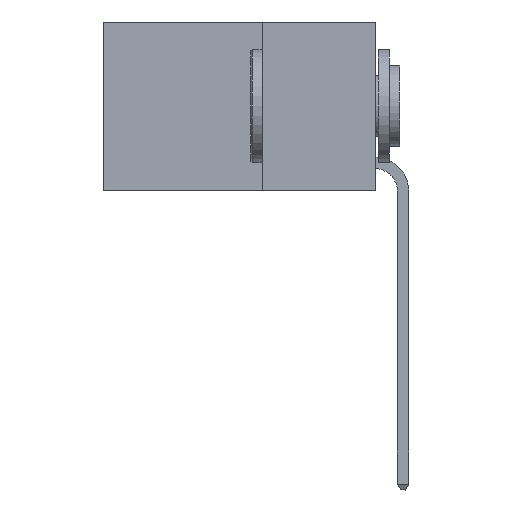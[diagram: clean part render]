
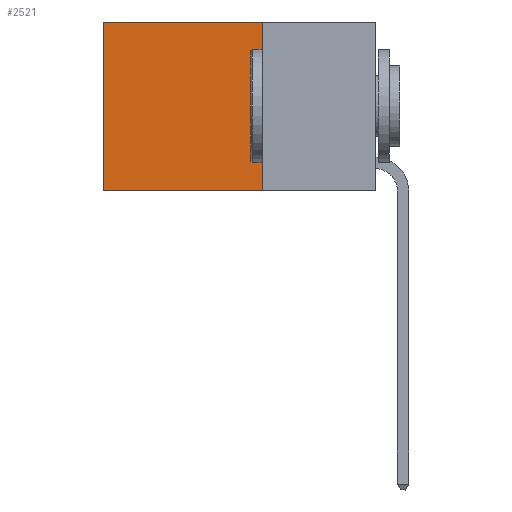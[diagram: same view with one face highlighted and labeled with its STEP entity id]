
A CAD part, left-side view. The second image highlights one B-rep face of the part: STEP entity #2521.
In plain terms, the highlighted planar face has unit normal (-1, 0, 0).
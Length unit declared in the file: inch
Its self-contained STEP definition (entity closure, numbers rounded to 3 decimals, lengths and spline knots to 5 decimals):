
#138 = DIRECTION ( 'NONE',  ( 1., 0., 0. ) ) ;
#178 = CARTESIAN_POINT ( 'NONE',  ( 0.2625, 0.25, 0. ) ) ;
#941 = EDGE_CURVE ( 'NONE', #2041, #2436, #18137, .T. ) ;
#1561 = VECTOR ( 'NONE', #4664, 39.37008 ) ;
#1666 = VECTOR ( 'NONE', #15368, 39.37008 ) ;
#2041 = VERTEX_POINT ( 'NONE', #15160 ) ;
#2043 = PLANE ( 'NONE',  #16522 ) ;
#2059 = EDGE_CURVE ( 'NONE', #6243, #9683, #5286, .T. ) ;
#2436 = VERTEX_POINT ( 'NONE', #14094 ) ;
#2521 = ADVANCED_FACE ( 'NONE', ( #11496 ), #2043, .F. ) ;
#2674 = EDGE_CURVE ( 'NONE', #9683, #2436, #8812, .T. ) ;
#2697 = ORIENTED_EDGE ( 'NONE', *, *, #2059, .F. ) ;
#4664 = DIRECTION ( 'NONE',  ( 0., 1., 0. ) ) ;
#5286 = LINE ( 'NONE', #14802, #15726 ) ;
#6228 = ORIENTED_EDGE ( 'NONE', *, *, #941, .T. ) ;
#6243 = VERTEX_POINT ( 'NONE', #6688 ) ;
#6688 = CARTESIAN_POINT ( 'NONE',  ( 0.2625, 0.25, 0. ) ) ;
#6843 = VECTOR ( 'NONE', #8736, 39.37008 ) ;
#8736 = DIRECTION ( 'NONE',  ( 0., 0., -1. ) ) ;
#8812 = LINE ( 'NONE', #16764, #1561 ) ;
#9165 = CARTESIAN_POINT ( 'NONE',  ( 0.2625, 0.6, 0. ) ) ;
#9364 = LINE ( 'NONE', #12589, #1666 ) ;
#9683 = VERTEX_POINT ( 'NONE', #11292 ) ;
#11292 = CARTESIAN_POINT ( 'NONE',  ( 0.2625, 0.25, -0.37 ) ) ;
#11496 = FACE_OUTER_BOUND ( 'NONE', #12925, .T. ) ;
#12589 = CARTESIAN_POINT ( 'NONE',  ( 0.2625, 0.25, 0. ) ) ;
#12925 = EDGE_LOOP ( 'NONE', ( #6228, #13029, #2697, #12973 ) ) ;
#12973 = ORIENTED_EDGE ( 'NONE', *, *, #17957, .T. ) ;
#13029 = ORIENTED_EDGE ( 'NONE', *, *, #2674, .F. ) ;
#14094 = CARTESIAN_POINT ( 'NONE',  ( 0.2625, 0.6, -0.37 ) ) ;
#14802 = CARTESIAN_POINT ( 'NONE',  ( 0.2625, 0.25, 0. ) ) ;
#15160 = CARTESIAN_POINT ( 'NONE',  ( 0.2625, 0.6, 0. ) ) ;
#15368 = DIRECTION ( 'NONE',  ( 0., 1., 0. ) ) ;
#15726 = VECTOR ( 'NONE', #16306, 39.37008 ) ;
#15764 = DIRECTION ( 'NONE',  ( 0., 0., -1. ) ) ;
#16306 = DIRECTION ( 'NONE',  ( 0., 0., -1. ) ) ;
#16522 = AXIS2_PLACEMENT_3D ( 'NONE', #178, #138, #15764 ) ;
#16764 = CARTESIAN_POINT ( 'NONE',  ( 0.2625, 0.25, -0.37 ) ) ;
#17957 = EDGE_CURVE ( 'NONE', #6243, #2041, #9364, .T. ) ;
#18137 = LINE ( 'NONE', #9165, #6843 ) ;
